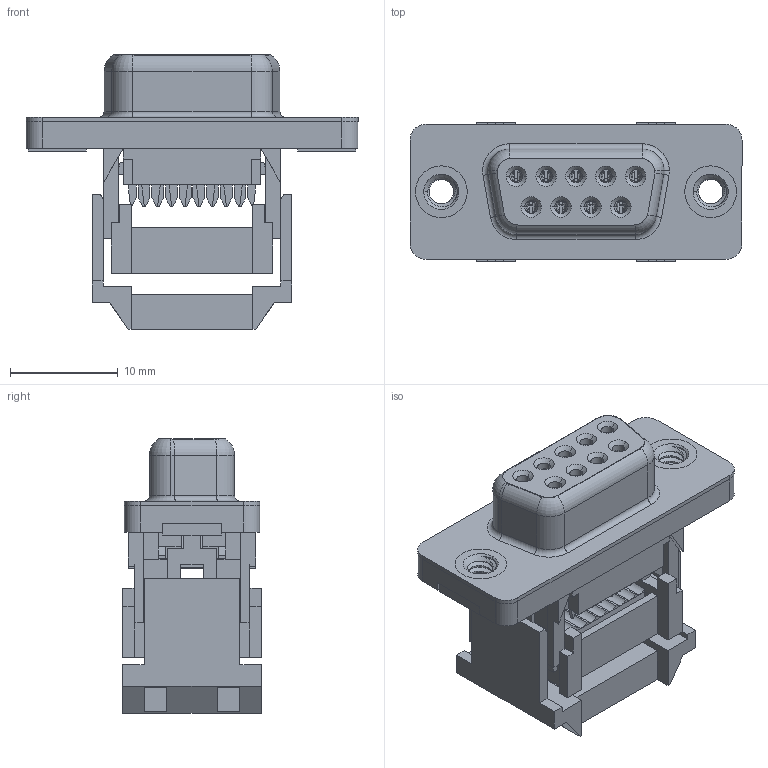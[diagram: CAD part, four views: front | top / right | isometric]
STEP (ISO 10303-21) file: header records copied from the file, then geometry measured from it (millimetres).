
FILE_DESCRIPTION (( 'STEP AP203' ), '1' );
FILE_NAME ('628-009-227-012.STEP', '2020-07-16T13:35:15', ( '' ), ( '' ), 'SwSTEP 2.0', 'SolidWorks 2020', '' );
FILE_SCHEMA (( 'CONFIG_CONTROL_DESIGN' ));
Length unit declared in the file: millimetre
Products named in the file (8): 628 IDC Cable Cover_09 Contacts; 628 IDC Guide Rear_09 Contacts; 628 IDC Guide Front_09 Contacts; 628 PB Shell_09 Contacts; 628 IDC Contacts_09 Contacts; 628-009-227-012; 628 IDC Housing_09 Contacts; 628 IDC 4-40 Threaded Rivet
Assembly tree (8 placements, depth 2):
  628-009-227-012
    628 IDC Housing_09 Contacts
    628 IDC Guide Front_09 Contacts
    628 IDC Guide Rear_09 Contacts
    628 IDC Cable Cover_09 Contacts
    628 PB Shell_09 Contacts
    628 IDC Contacts_09 Contacts
    628 IDC 4-40 Threaded Rivet  x2
Bounding box: 30.81 x 12.85 x 25.5 mm (x, y, z)
Volume: 3148.6 mm3; surface area: 6642 mm2
Topology: 18 solids, 18 shells, 1783 faces, 4575 edges, 2850 vertices
Faces by surface type: plane 1112, cylinder 363, torus 175, cone 118, bspline 15
Entity records: 54998 total; most frequent: CARTESIAN_POINT 11022, DIRECTION 9027, ORIENTED_EDGE 9000, EDGE_CURVE 4500, VECTOR 3271, LINE 3271, AXIS2_PLACEMENT_3D 2878, VERTEX_POINT 2801
